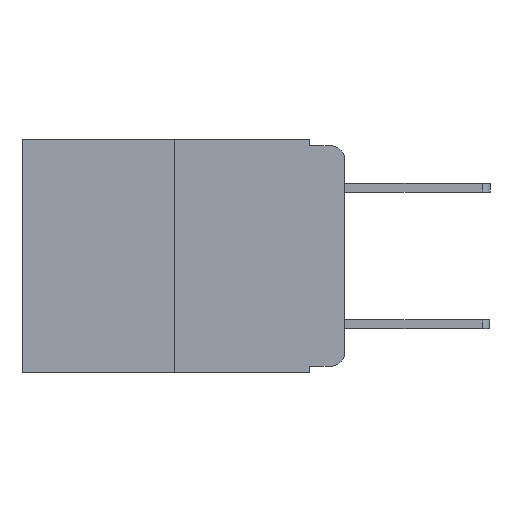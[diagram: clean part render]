
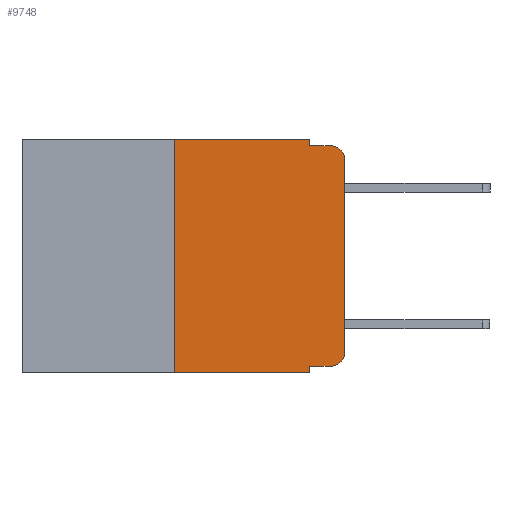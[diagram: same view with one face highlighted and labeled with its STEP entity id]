
A CAD part, left-side view. The second image highlights one B-rep face of the part: STEP entity #9748.
In plain terms, the highlighted planar face has unit normal (-1, 0, 0).
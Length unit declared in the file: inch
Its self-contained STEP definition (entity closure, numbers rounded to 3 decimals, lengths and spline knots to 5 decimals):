
#411 = CARTESIAN_POINT ( 'NONE',  ( 0., 0.051, -0.343 ) ) ;
#431 = AXIS2_PLACEMENT_3D ( 'NONE', #18566, #18693, #18717 ) ;
#665 = VERTEX_POINT ( 'NONE', #3076 ) ;
#689 = PLANE ( 'NONE',  #17749 ) ;
#1003 = CARTESIAN_POINT ( 'NONE',  ( 0., 0.25, 0. ) ) ;
#1286 = ORIENTED_EDGE ( 'NONE', *, *, #18649, .T. ) ;
#1396 = EDGE_CURVE ( 'NONE', #12288, #1624, #19175, .T. ) ;
#1624 = VERTEX_POINT ( 'NONE', #411 ) ;
#2378 = DIRECTION ( 'NONE',  ( 0., 0., -1. ) ) ;
#2438 = ORIENTED_EDGE ( 'NONE', *, *, #3346, .F. ) ;
#3076 = CARTESIAN_POINT ( 'NONE',  ( 0., 0.25, -0.343 ) ) ;
#3129 = ORIENTED_EDGE ( 'NONE', *, *, #18809, .T. ) ;
#3171 = ORIENTED_EDGE ( 'NONE', *, *, #3662, .T. ) ;
#3346 = EDGE_CURVE ( 'NONE', #8148, #13919, #8026, .T. ) ;
#3662 = EDGE_CURVE ( 'NONE', #12288, #9475, #6125, .T. ) ;
#3962 = DIRECTION ( 'NONE',  ( 0., 0., 1. ) ) ;
#3988 = DIRECTION ( 'NONE',  ( 0., -1., 0. ) ) ;
#4958 = CARTESIAN_POINT ( 'NONE',  ( 0., 0.02, -0.333 ) ) ;
#4988 = DIRECTION ( 'NONE',  ( 0., 0., -1. ) ) ;
#5795 = ORIENTED_EDGE ( 'NONE', *, *, #1396, .F. ) ;
#6051 = EDGE_CURVE ( 'NONE', #665, #8148, #7115, .T. ) ;
#6125 = LINE ( 'NONE', #13878, #10072 ) ;
#6173 = CARTESIAN_POINT ( 'NONE',  ( 0., 0.051, -0.01 ) ) ;
#6392 = LINE ( 'NONE', #17361, #19194 ) ;
#6531 = CIRCLE ( 'NONE', #431, 0.02 ) ;
#6674 = CARTESIAN_POINT ( 'NONE',  ( 0., 0.051, -0.333 ) ) ;
#6941 = EDGE_CURVE ( 'NONE', #8874, #7448, #6531, .T. ) ;
#7115 = LINE ( 'NONE', #1003, #15504 ) ;
#7448 = VERTEX_POINT ( 'NONE', #18474 ) ;
#7662 = CARTESIAN_POINT ( 'NONE',  ( 0., 0.02, -0.313 ) ) ;
#7941 = ORIENTED_EDGE ( 'NONE', *, *, #6051, .F. ) ;
#8026 = LINE ( 'NONE', #11781, #16379 ) ;
#8148 = VERTEX_POINT ( 'NONE', #13297 ) ;
#8620 = DIRECTION ( 'NONE',  ( 0., -1., 0. ) ) ;
#8874 = VERTEX_POINT ( 'NONE', #20060 ) ;
#8892 = AXIS2_PLACEMENT_3D ( 'NONE', #7662, #19300, #9340 ) ;
#9340 = DIRECTION ( 'NONE',  ( 0., 0., -1. ) ) ;
#9344 = EDGE_LOOP ( 'NONE', ( #3129, #13869, #19179, #20444, #2438, #7941, #1286, #5795, #3171, #19099 ) ) ;
#9475 = VERTEX_POINT ( 'NONE', #4958 ) ;
#9748 = ADVANCED_FACE ( 'NONE', ( #11130 ), #689, .F. ) ;
#10072 = VECTOR ( 'NONE', #13294, 39.37008 ) ;
#10185 = CARTESIAN_POINT ( 'NONE',  ( 0., 0.473, -0.343 ) ) ;
#11130 = FACE_OUTER_BOUND ( 'NONE', #9344, .T. ) ;
#11781 = CARTESIAN_POINT ( 'NONE',  ( 0., 0.473, 0. ) ) ;
#12179 = DIRECTION ( 'NONE',  ( 0., -1., 0. ) ) ;
#12288 = VERTEX_POINT ( 'NONE', #6674 ) ;
#12309 = CARTESIAN_POINT ( 'NONE',  ( 0., 0., 0. ) ) ;
#12431 = DIRECTION ( 'NONE',  ( 1., 0., 0. ) ) ;
#13023 = CARTESIAN_POINT ( 'NONE',  ( 0., 0., -0.313 ) ) ;
#13294 = DIRECTION ( 'NONE',  ( 0., -1., 0. ) ) ;
#13297 = CARTESIAN_POINT ( 'NONE',  ( 0., 0.25, 0. ) ) ;
#13651 = VERTEX_POINT ( 'NONE', #6173 ) ;
#13857 = LINE ( 'NONE', #16996, #17744 ) ;
#13869 = ORIENTED_EDGE ( 'NONE', *, *, #6941, .T. ) ;
#13878 = CARTESIAN_POINT ( 'NONE',  ( 0., 0.051, -0.333 ) ) ;
#13919 = VERTEX_POINT ( 'NONE', #16854 ) ;
#14228 = EDGE_CURVE ( 'NONE', #9475, #17276, #21252, .T. ) ;
#14764 = VECTOR ( 'NONE', #8620, 39.37008 ) ;
#15504 = VECTOR ( 'NONE', #18652, 39.37008 ) ;
#15822 = VECTOR ( 'NONE', #4988, 39.37008 ) ;
#16074 = VECTOR ( 'NONE', #3962, 39.37008 ) ;
#16379 = VECTOR ( 'NONE', #12179, 39.37008 ) ;
#16854 = CARTESIAN_POINT ( 'NONE',  ( 0., 0.051, 0. ) ) ;
#16996 = CARTESIAN_POINT ( 'NONE',  ( 0., 0.051, 0. ) ) ;
#17276 = VERTEX_POINT ( 'NONE', #13023 ) ;
#17361 = CARTESIAN_POINT ( 'NONE',  ( 0., 0.051, -0.01 ) ) ;
#17744 = VECTOR ( 'NONE', #18655, 39.37008 ) ;
#17749 = AXIS2_PLACEMENT_3D ( 'NONE', #19038, #12431, #2378 ) ;
#18221 = EDGE_CURVE ( 'NONE', #13651, #7448, #6392, .T. ) ;
#18474 = CARTESIAN_POINT ( 'NONE',  ( 0., 0.02, -0.01 ) ) ;
#18566 = CARTESIAN_POINT ( 'NONE',  ( 0., 0.02, -0.03 ) ) ;
#18649 = EDGE_CURVE ( 'NONE', #665, #1624, #19172, .T. ) ;
#18652 = DIRECTION ( 'NONE',  ( 0., 0., 1. ) ) ;
#18655 = DIRECTION ( 'NONE',  ( 0., 0., -1. ) ) ;
#18693 = DIRECTION ( 'NONE',  ( -1., 0., 0. ) ) ;
#18717 = DIRECTION ( 'NONE',  ( 0., 0., -1. ) ) ;
#18809 = EDGE_CURVE ( 'NONE', #17276, #8874, #20938, .T. ) ;
#19038 = CARTESIAN_POINT ( 'NONE',  ( 0., 0.473, 0. ) ) ;
#19099 = ORIENTED_EDGE ( 'NONE', *, *, #14228, .T. ) ;
#19172 = LINE ( 'NONE', #10185, #14764 ) ;
#19175 = LINE ( 'NONE', #19772, #15822 ) ;
#19179 = ORIENTED_EDGE ( 'NONE', *, *, #18221, .F. ) ;
#19194 = VECTOR ( 'NONE', #3988, 39.37008 ) ;
#19300 = DIRECTION ( 'NONE',  ( -1., 0., 0. ) ) ;
#19772 = CARTESIAN_POINT ( 'NONE',  ( 0., 0.051, 0. ) ) ;
#20060 = CARTESIAN_POINT ( 'NONE',  ( 0., 0., -0.03 ) ) ;
#20444 = ORIENTED_EDGE ( 'NONE', *, *, #21207, .F. ) ;
#20938 = LINE ( 'NONE', #12309, #16074 ) ;
#21207 = EDGE_CURVE ( 'NONE', #13919, #13651, #13857, .T. ) ;
#21252 = CIRCLE ( 'NONE', #8892, 0.02 ) ;
